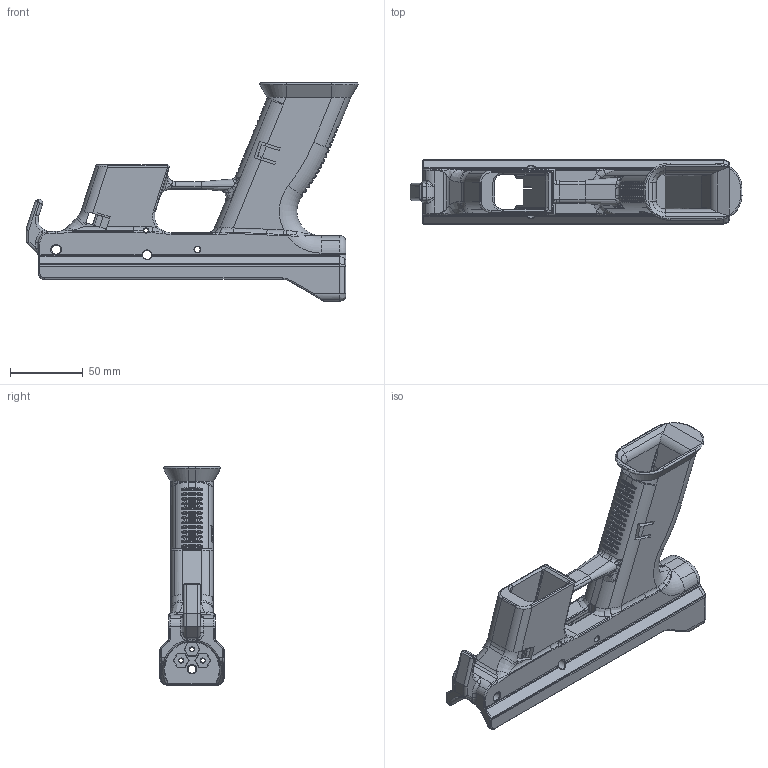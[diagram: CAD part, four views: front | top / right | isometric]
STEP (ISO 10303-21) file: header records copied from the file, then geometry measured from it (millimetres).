
FILE_DESCRIPTION (( 'STEP AP203' ), '1' );
FILE_NAME ('GAB-10_V4.STEP', '2020-02-07T01:25:24', ( '' ), ( '' ), 'SwSTEP 2.0', 'SolidWorks 2019', '' );
FILE_SCHEMA (( 'CONFIG_CONTROL_DESIGN' ));
Length unit declared in the file: millimetre
Products named in the file (1): GAB-10_V4
Bounding box: 227.94 x 44 x 149.96 mm (x, y, z)
Volume: 244039.3 mm3; surface area: 84872.6 mm2
Topology: 1 solids, 1 shells, 1271 faces, 3228 edges, 1917 vertices
Faces by surface type: cylinder 496, bspline 394, plane 246, torus 83, cone 50, sphere 2
Entity records: 54170 total; most frequent: CARTESIAN_POINT 27797, ORIENTED_EDGE 6400, DIRECTION 4019, EDGE_CURVE 3200, VERTEX_POINT 1917, AXIS2_PLACEMENT_3D 1438, B_SPLINE_CURVE_WITH_KNOTS 1376, EDGE_LOOP 1293
